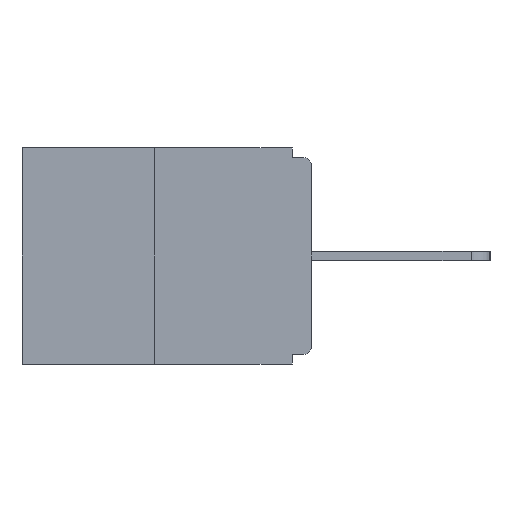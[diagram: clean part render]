
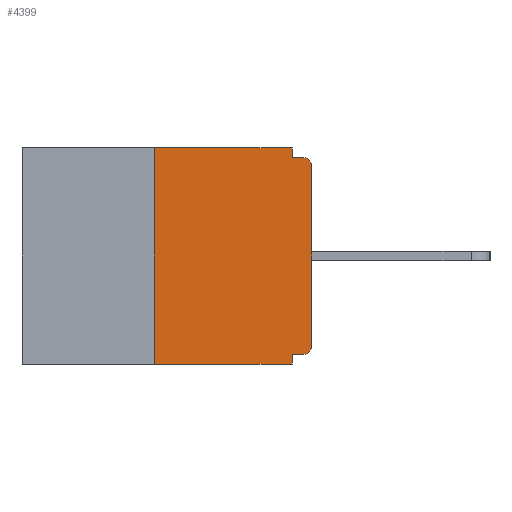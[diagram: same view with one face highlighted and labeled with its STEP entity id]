
A CAD part, left-side view. The second image highlights one B-rep face of the part: STEP entity #4399.
In plain terms, the highlighted planar face has unit normal (-1, 0, 0).
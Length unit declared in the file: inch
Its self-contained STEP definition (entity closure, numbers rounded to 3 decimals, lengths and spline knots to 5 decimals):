
#280 = CARTESIAN_POINT ( 'NONE',  ( 0., 0.46, 0. ) ) ;
#384 = PLANE ( 'NONE',  #4908 ) ;
#638 = CARTESIAN_POINT ( 'NONE',  ( 0., 0.031, 0. ) ) ;
#720 = CIRCLE ( 'NONE', #20783, 0.015 ) ;
#900 = LINE ( 'NONE', #7313, #13832 ) ;
#1066 = CARTESIAN_POINT ( 'NONE',  ( 0., 0., -0.015 ) ) ;
#1233 = DIRECTION ( 'NONE',  ( 0., -1., 0. ) ) ;
#1839 = VECTOR ( 'NONE', #5957, 39.37008 ) ;
#2045 = VECTOR ( 'NONE', #5177, 39.37008 ) ;
#2185 = VECTOR ( 'NONE', #22087, 39.37008 ) ;
#2508 = EDGE_CURVE ( 'NONE', #8997, #3415, #900, .T. ) ;
#2556 = CARTESIAN_POINT ( 'NONE',  ( 0., 0.031, -0.328 ) ) ;
#2773 = VECTOR ( 'NONE', #21728, 39.37008 ) ;
#2949 = CARTESIAN_POINT ( 'NONE',  ( 0., 0.031, -0.343 ) ) ;
#3415 = VERTEX_POINT ( 'NONE', #2949 ) ;
#3709 = EDGE_CURVE ( 'NONE', #10072, #16760, #15857, .T. ) ;
#3886 = CARTESIAN_POINT ( 'NONE',  ( 0., 0.015, -0.313 ) ) ;
#4399 = ADVANCED_FACE ( 'NONE', ( #5879 ), #384, .F. ) ;
#4598 = CARTESIAN_POINT ( 'NONE',  ( 0., 0.25, -0.343 ) ) ;
#4707 = LINE ( 'NONE', #5027, #22358 ) ;
#4708 = CARTESIAN_POINT ( 'NONE',  ( 0., 0., 0. ) ) ;
#4891 = CARTESIAN_POINT ( 'NONE',  ( 0., 0.031, -0.015 ) ) ;
#4908 = AXIS2_PLACEMENT_3D ( 'NONE', #280, #16647, #6704 ) ;
#5027 = CARTESIAN_POINT ( 'NONE',  ( 0., 0., -0.328 ) ) ;
#5151 = VERTEX_POINT ( 'NONE', #2556 ) ;
#5177 = DIRECTION ( 'NONE',  ( 0., 0., -1. ) ) ;
#5676 = DIRECTION ( 'NONE',  ( 0., 0., -1. ) ) ;
#5879 = FACE_OUTER_BOUND ( 'NONE', #9106, .T. ) ;
#5957 = DIRECTION ( 'NONE',  ( 0., 0., 1. ) ) ;
#6067 = EDGE_CURVE ( 'NONE', #8997, #15814, #11232, .T. ) ;
#6704 = DIRECTION ( 'NONE',  ( 0., 0., -1. ) ) ;
#7313 = CARTESIAN_POINT ( 'NONE',  ( 0., 0.46, -0.343 ) ) ;
#8410 = CIRCLE ( 'NONE', #11930, 0.015 ) ;
#8564 = LINE ( 'NONE', #1066, #2773 ) ;
#8997 = VERTEX_POINT ( 'NONE', #4598 ) ;
#9036 = EDGE_CURVE ( 'NONE', #15814, #10072, #21073, .T. ) ;
#9106 = EDGE_LOOP ( 'NONE', ( #11099, #19265, #10366, #9341, #19312, #14244, #17977, #21150, #14901, #20998 ) ) ;
#9153 = CARTESIAN_POINT ( 'NONE',  ( 0., 0.015, -0.03 ) ) ;
#9341 = ORIENTED_EDGE ( 'NONE', *, *, #17238, .F. ) ;
#10072 = VERTEX_POINT ( 'NONE', #19942 ) ;
#10360 = DIRECTION ( 'NONE',  ( 0., 1., 0. ) ) ;
#10366 = ORIENTED_EDGE ( 'NONE', *, *, #2508, .T. ) ;
#10497 = EDGE_CURVE ( 'NONE', #15062, #16484, #720, .T. ) ;
#10945 = DIRECTION ( 'NONE',  ( 0., 0., -1. ) ) ;
#11099 = ORIENTED_EDGE ( 'NONE', *, *, #9036, .F. ) ;
#11232 = LINE ( 'NONE', #20506, #1839 ) ;
#11263 = VERTEX_POINT ( 'NONE', #19519 ) ;
#11803 = CARTESIAN_POINT ( 'NONE',  ( 0., 0.46, 0. ) ) ;
#11930 = AXIS2_PLACEMENT_3D ( 'NONE', #3886, #15971, #5676 ) ;
#11932 = EDGE_CURVE ( 'NONE', #18213, #11263, #8410, .T. ) ;
#12130 = VECTOR ( 'NONE', #16766, 39.37008 ) ;
#12850 = CARTESIAN_POINT ( 'NONE',  ( 0., 0.015, -0.015 ) ) ;
#13734 = CARTESIAN_POINT ( 'NONE',  ( 0., 0.031, -0.343 ) ) ;
#13832 = VECTOR ( 'NONE', #19513, 39.37008 ) ;
#13920 = EDGE_CURVE ( 'NONE', #11263, #15062, #16071, .T. ) ;
#13928 = CARTESIAN_POINT ( 'NONE',  ( 0., 0., -0.03 ) ) ;
#14052 = EDGE_CURVE ( 'NONE', #18213, #5151, #4707, .T. ) ;
#14244 = ORIENTED_EDGE ( 'NONE', *, *, #11932, .T. ) ;
#14336 = CARTESIAN_POINT ( 'NONE',  ( 0., 0.25, 0. ) ) ;
#14901 = ORIENTED_EDGE ( 'NONE', *, *, #21651, .F. ) ;
#15062 = VERTEX_POINT ( 'NONE', #13928 ) ;
#15814 = VERTEX_POINT ( 'NONE', #14336 ) ;
#15857 = LINE ( 'NONE', #638, #2045 ) ;
#15971 = DIRECTION ( 'NONE',  ( -1., 0., 0. ) ) ;
#16071 = LINE ( 'NONE', #4708, #12130 ) ;
#16484 = VERTEX_POINT ( 'NONE', #12850 ) ;
#16587 = VECTOR ( 'NONE', #1233, 39.37008 ) ;
#16647 = DIRECTION ( 'NONE',  ( 1., 0., 0. ) ) ;
#16760 = VERTEX_POINT ( 'NONE', #4891 ) ;
#16766 = DIRECTION ( 'NONE',  ( 0., 0., 1. ) ) ;
#17238 = EDGE_CURVE ( 'NONE', #5151, #3415, #20487, .T. ) ;
#17977 = ORIENTED_EDGE ( 'NONE', *, *, #13920, .T. ) ;
#18213 = VERTEX_POINT ( 'NONE', #21628 ) ;
#19265 = ORIENTED_EDGE ( 'NONE', *, *, #6067, .F. ) ;
#19312 = ORIENTED_EDGE ( 'NONE', *, *, #14052, .F. ) ;
#19513 = DIRECTION ( 'NONE',  ( 0., -1., 0. ) ) ;
#19519 = CARTESIAN_POINT ( 'NONE',  ( 0., 0., -0.313 ) ) ;
#19942 = CARTESIAN_POINT ( 'NONE',  ( 0., 0.031, 0. ) ) ;
#20487 = LINE ( 'NONE', #13734, #2185 ) ;
#20506 = CARTESIAN_POINT ( 'NONE',  ( 0., 0.25, 0. ) ) ;
#20783 = AXIS2_PLACEMENT_3D ( 'NONE', #9153, #21011, #10945 ) ;
#20998 = ORIENTED_EDGE ( 'NONE', *, *, #3709, .F. ) ;
#21011 = DIRECTION ( 'NONE',  ( -1., 0., 0. ) ) ;
#21073 = LINE ( 'NONE', #11803, #16587 ) ;
#21150 = ORIENTED_EDGE ( 'NONE', *, *, #10497, .T. ) ;
#21628 = CARTESIAN_POINT ( 'NONE',  ( 0., 0.015, -0.328 ) ) ;
#21651 = EDGE_CURVE ( 'NONE', #16760, #16484, #8564, .T. ) ;
#21728 = DIRECTION ( 'NONE',  ( 0., -1., 0. ) ) ;
#22087 = DIRECTION ( 'NONE',  ( 0., 0., -1. ) ) ;
#22358 = VECTOR ( 'NONE', #10360, 39.37008 ) ;
